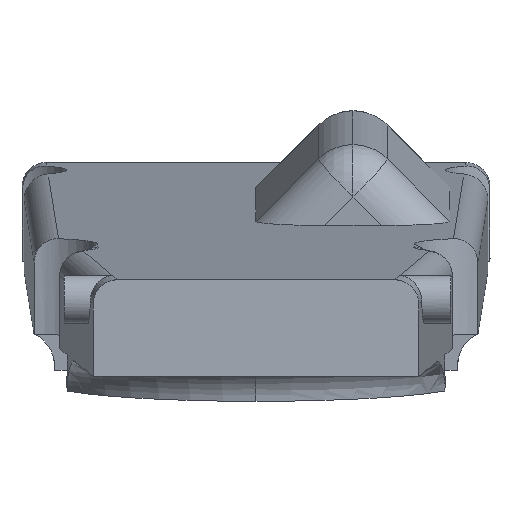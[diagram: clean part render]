
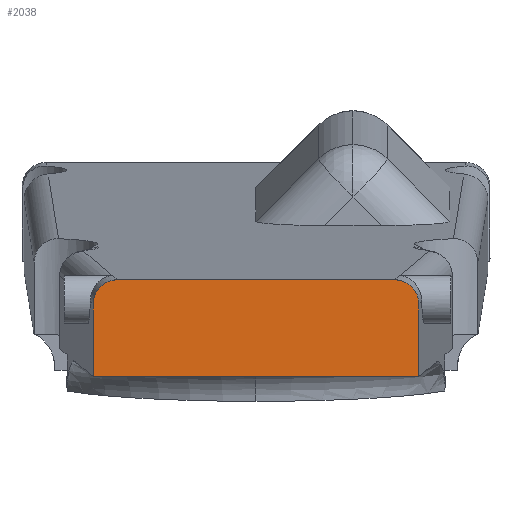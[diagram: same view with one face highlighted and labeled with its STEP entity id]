
A CAD part, left-side view. The second image highlights one B-rep face of the part: STEP entity #2038.
In plain terms, the highlighted planar face has unit normal (-1, 0, 0).
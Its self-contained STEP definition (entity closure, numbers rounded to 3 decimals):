
#120 = ORIENTED_EDGE ( 'NONE', *, *, #1001, .T. ) ;
#195 = ORIENTED_EDGE ( 'NONE', *, *, #1166, .T. ) ;
#262 = CARTESIAN_POINT ( 'NONE',  ( -72.873, -7.265, 62. ) ) ;
#378 = CARTESIAN_POINT ( 'NONE',  ( -72.873, 7.336, 62. ) ) ;
#384 = CARTESIAN_POINT ( 'NONE',  ( -72.873, 8.53, 61.384 ) ) ;
#460 = VECTOR ( 'NONE', #2007, 1000. ) ;
#576 = VERTEX_POINT ( 'NONE', #2741 ) ;
#578 = CARTESIAN_POINT ( 'NONE',  ( -72.873, -7.475, 61.983 ) ) ;
#586 = CARTESIAN_POINT ( 'NONE',  ( -72.873, 7.476, 61.983 ) ) ;
#646 = DIRECTION ( 'NONE',  ( 1., 0., 0. ) ) ;
#670 = VERTEX_POINT ( 'NONE', #262 ) ;
#955 = VERTEX_POINT ( 'NONE', #1802 ) ;
#968 = CARTESIAN_POINT ( 'NONE',  ( -72.873, -8.53, 56.92 ) ) ;
#1001 = EDGE_CURVE ( 'NONE', #670, #1031, #1053, .T. ) ;
#1010 = EDGE_CURVE ( 'NONE', #1380, #2639, #2134, .T. ) ;
#1031 = VERTEX_POINT ( 'NONE', #1395 ) ;
#1053 = LINE ( 'NONE', #2745, #460 ) ;
#1110 = CARTESIAN_POINT ( 'NONE',  ( -72.873, -11.536, 60.737 ) ) ;
#1166 = EDGE_CURVE ( 'NONE', #2385, #1380, #2435, .T. ) ;
#1198 = DIRECTION ( 'NONE',  ( 0., 0., 1. ) ) ;
#1199 = EDGE_CURVE ( 'NONE', #2639, #955, #1211, .T. ) ;
#1211 = LINE ( 'NONE', #2034, #2255 ) ;
#1246 = EDGE_CURVE ( 'NONE', #955, #2003, #2662, .T. ) ;
#1250 = EDGE_CURVE ( 'NONE', #2003, #670, #2236, .T. ) ;
#1253 = ORIENTED_EDGE ( 'NONE', *, *, #1010, .T. ) ;
#1257 = EDGE_CURVE ( 'NONE', #1031, #576, #1815, .T. ) ;
#1265 = EDGE_CURVE ( 'NONE', #576, #2385, #1267, .T. ) ;
#1267 =( BOUNDED_CURVE ( )  B_SPLINE_CURVE ( 3, ( #1544, #1776, #384, #1956 ),
 .UNSPECIFIED., .F., .T. ) 
 B_SPLINE_CURVE_WITH_KNOTS ( ( 4, 4 ),
 ( 5.585, 6.981 ),
 .UNSPECIFIED. ) 
 CURVE ( )  GEOMETRIC_REPRESENTATION_ITEM ( )  RATIONAL_B_SPLINE_CURVE ( ( 1., 0.844, 0.844, 1. ) ) 
 REPRESENTATION_ITEM ( '' )  );
#1274 = CARTESIAN_POINT ( 'NONE',  ( -72.873, -8.114, 61.876 ) ) ;
#1284 = CARTESIAN_POINT ( 'NONE',  ( -72.873, -7.336, 62. ) ) ;
#1333 = ORIENTED_EDGE ( 'NONE', *, *, #1257, .T. ) ;
#1340 = CARTESIAN_POINT ( 'NONE',  ( -72.873, 8.53, -70.796 ) ) ;
#1358 = DIRECTION ( 'NONE',  ( 0., 0., -1. ) ) ;
#1380 = VERTEX_POINT ( 'NONE', #1633 ) ;
#1395 = CARTESIAN_POINT ( 'NONE',  ( -72.873, 7.265, 62. ) ) ;
#1496 = CARTESIAN_POINT ( 'NONE',  ( -72.873, -8.53, 60.737 ) ) ;
#1516 = FACE_OUTER_BOUND ( 'NONE', #2203, .T. ) ;
#1544 = CARTESIAN_POINT ( 'NONE',  ( -72.873, 7.476, 61.983 ) ) ;
#1633 = CARTESIAN_POINT ( 'NONE',  ( -72.873, 8.53, 56.92 ) ) ;
#1643 = ORIENTED_EDGE ( 'NONE', *, *, #1246, .T. ) ;
#1762 = CARTESIAN_POINT ( 'NONE',  ( -72.873, 7.265, 62. ) ) ;
#1776 = CARTESIAN_POINT ( 'NONE',  ( -72.873, 8.114, 61.876 ) ) ;
#1802 = CARTESIAN_POINT ( 'NONE',  ( -72.873, -8.53, 60.737 ) ) ;
#1815 = B_SPLINE_CURVE_WITH_KNOTS ( 'NONE', 3,
 ( #1762, #378, #1948, #586 ),
 .UNSPECIFIED., .F., .F.,
 ( 4, 4 ),
 ( 0., 0. ),
 .UNSPECIFIED. ) ;
#1865 = ORIENTED_EDGE ( 'NONE', *, *, #1199, .T. ) ;
#1916 = ORIENTED_EDGE ( 'NONE', *, *, #1265, .T. ) ;
#1938 = VECTOR ( 'NONE', #2723, 1000. ) ;
#1939 = CARTESIAN_POINT ( 'NONE',  ( -72.873, -7.406, 61.995 ) ) ;
#1948 = CARTESIAN_POINT ( 'NONE',  ( -72.873, 7.406, 61.995 ) ) ;
#1956 = CARTESIAN_POINT ( 'NONE',  ( -72.873, 8.53, 60.737 ) ) ;
#2003 = VERTEX_POINT ( 'NONE', #2736 ) ;
#2007 = DIRECTION ( 'NONE',  ( 0., 1., 0. ) ) ;
#2034 = CARTESIAN_POINT ( 'NONE',  ( -72.873, -8.53, 66.864 ) ) ;
#2038 = ADVANCED_FACE ( 'NONE', ( #1516 ), #2374, .F. ) ;
#2100 = CARTESIAN_POINT ( 'NONE',  ( -72.873, -8.53, 61.384 ) ) ;
#2134 = LINE ( 'NONE', #2393, #2580 ) ;
#2203 = EDGE_LOOP ( 'NONE', ( #1253, #1865, #1643, #2360, #120, #1333, #1916, #195 ) ) ;
#2236 = B_SPLINE_CURVE_WITH_KNOTS ( 'NONE', 3,
 ( #578, #1939, #1284, #2679 ),
 .UNSPECIFIED., .F., .F.,
 ( 4, 4 ),
 ( 0., 0. ),
 .UNSPECIFIED. ) ;
#2255 = VECTOR ( 'NONE', #1198, 1000. ) ;
#2360 = ORIENTED_EDGE ( 'NONE', *, *, #1250, .T. ) ;
#2374 = PLANE ( 'NONE',  #2478 ) ;
#2385 = VERTEX_POINT ( 'NONE', #2423 ) ;
#2393 = CARTESIAN_POINT ( 'NONE',  ( -72.873, 37.251, 56.92 ) ) ;
#2423 = CARTESIAN_POINT ( 'NONE',  ( -72.873, 8.53, 60.737 ) ) ;
#2435 = LINE ( 'NONE', #1340, #1938 ) ;
#2478 = AXIS2_PLACEMENT_3D ( 'NONE', #1110, #646, #1358 ) ;
#2571 = DIRECTION ( 'NONE',  ( 0., -1., 0. ) ) ;
#2580 = VECTOR ( 'NONE', #2571, 1000. ) ;
#2639 = VERTEX_POINT ( 'NONE', #968 ) ;
#2662 =( BOUNDED_CURVE ( )  B_SPLINE_CURVE ( 3, ( #1496, #2100, #1274, #2674 ),
 .UNSPECIFIED., .F., .T. ) 
 B_SPLINE_CURVE_WITH_KNOTS ( ( 4, 4 ),
 ( 2.444, 3.84 ),
 .UNSPECIFIED. ) 
 CURVE ( )  GEOMETRIC_REPRESENTATION_ITEM ( )  RATIONAL_B_SPLINE_CURVE ( ( 1., 0.844, 0.844, 1. ) ) 
 REPRESENTATION_ITEM ( '' )  );
#2674 = CARTESIAN_POINT ( 'NONE',  ( -72.873, -7.475, 61.983 ) ) ;
#2679 = CARTESIAN_POINT ( 'NONE',  ( -72.873, -7.265, 62. ) ) ;
#2723 = DIRECTION ( 'NONE',  ( 0., 0., -1. ) ) ;
#2736 = CARTESIAN_POINT ( 'NONE',  ( -72.873, -7.475, 61.983 ) ) ;
#2741 = CARTESIAN_POINT ( 'NONE',  ( -72.873, 7.476, 61.983 ) ) ;
#2745 = CARTESIAN_POINT ( 'NONE',  ( -72.873, 37.251, 62. ) ) ;
